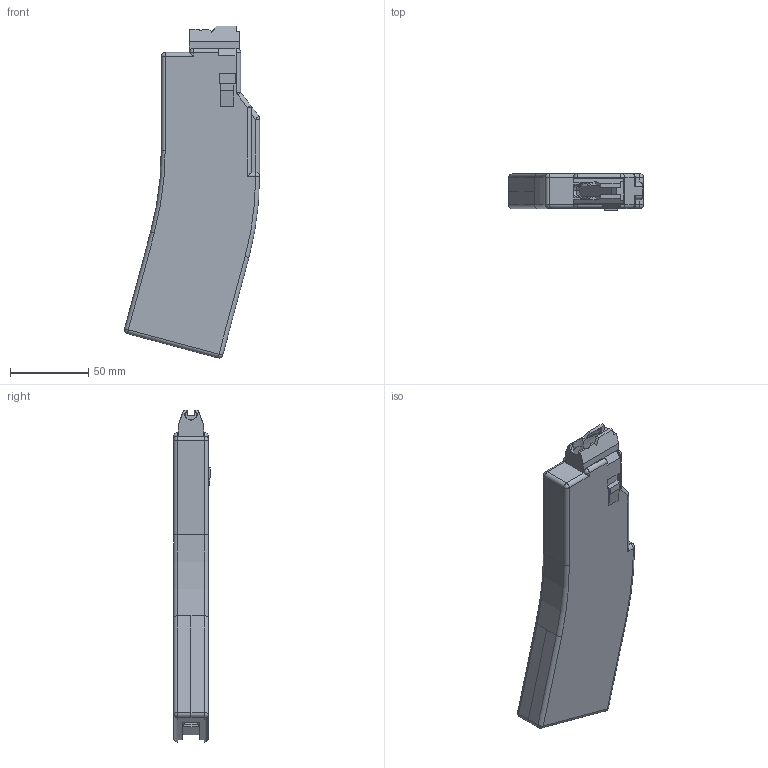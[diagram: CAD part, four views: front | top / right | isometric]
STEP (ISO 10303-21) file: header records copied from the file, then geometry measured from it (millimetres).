
FILE_DESCRIPTION(/* description */ (''),/* implementation_level */ '2;1');
FILE_NAME(/* name */ 'S&W15-22 Mag Solid Body.step',/* time_stamp */ '2021-06-26T18:16:54-06:00',/* author */ (''),/* organization */ (''),/* preprocessor_version */ 'ST-DEVELOPER v18.1',/* originating_system */ 'Autodesk Translation Framework v10.9.0.1377',/* authorisation */ '');
FILE_SCHEMA (('AUTOMOTIVE_DESIGN { 1 0 10303 214 3 1 1 }'));
Length unit declared in the file: millimetre
Products named in the file (1): S&W15-22 mag
Bounding box: 86.24 x 23.62 x 211.97 mm (x, y, z)
Volume: 215509.6 mm3; surface area: 49916.2 mm2
Topology: 1 solids, 1 shells, 291 faces, 737 edges, 442 vertices
Faces by surface type: plane 113, bspline 100, cylinder 65, sphere 9, torus 4
Entity records: 11783 total; most frequent: CARTESIAN_POINT 5377, ORIENTED_EDGE 1462, DIRECTION 1128, EDGE_CURVE 731, VERTEX_POINT 442, AXIS2_PLACEMENT_3D 417, LINE 294, VECTOR 294
